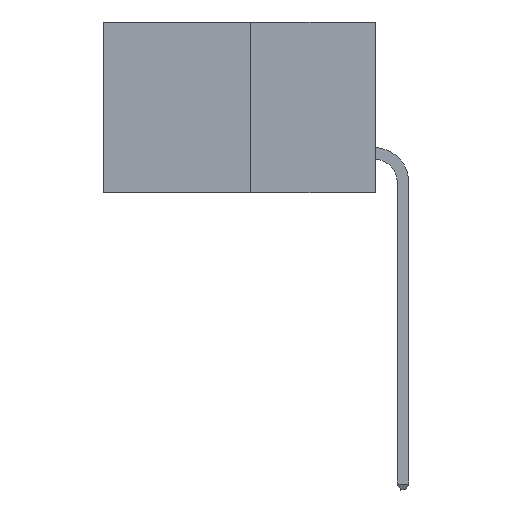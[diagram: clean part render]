
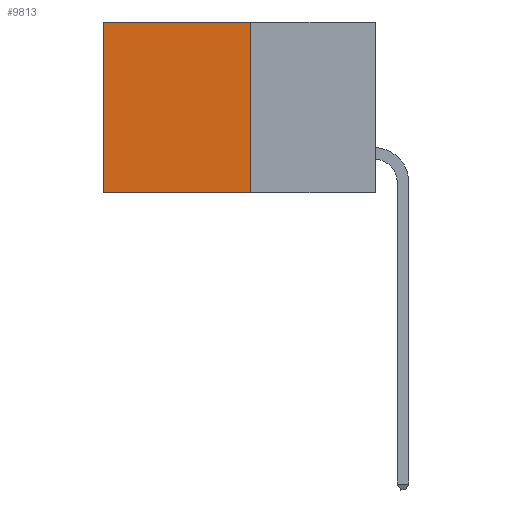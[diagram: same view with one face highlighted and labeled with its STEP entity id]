
A CAD part, left-side view. The second image highlights one B-rep face of the part: STEP entity #9813.
In plain terms, the highlighted planar face has unit normal (-1, 0, 0).
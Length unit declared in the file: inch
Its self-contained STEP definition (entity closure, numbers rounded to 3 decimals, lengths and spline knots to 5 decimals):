
#267 = CARTESIAN_POINT ( 'NONE',  ( 0.277, 0.27, 0. ) ) ;
#365 = ORIENTED_EDGE ( 'NONE', *, *, #638, .F. ) ;
#592 = CARTESIAN_POINT ( 'NONE',  ( 0.277, 0.27, -0.37 ) ) ;
#638 = EDGE_CURVE ( 'NONE', #8332, #10206, #4727, .T. ) ;
#952 = CARTESIAN_POINT ( 'NONE',  ( 0.277, 0.27, -0.37 ) ) ;
#1009 = DIRECTION ( 'NONE',  ( 0., 0., -1. ) ) ;
#1512 = VECTOR ( 'NONE', #13848, 39.37008 ) ;
#1978 = EDGE_LOOP ( 'NONE', ( #10787, #11857, #365, #2733 ) ) ;
#2433 = VECTOR ( 'NONE', #6500, 39.37008 ) ;
#2733 = ORIENTED_EDGE ( 'NONE', *, *, #5986, .T. ) ;
#3197 = VECTOR ( 'NONE', #8444, 39.37008 ) ;
#4685 = AXIS2_PLACEMENT_3D ( 'NONE', #952, #7976, #1009 ) ;
#4727 = LINE ( 'NONE', #12705, #1512 ) ;
#4744 = CARTESIAN_POINT ( 'NONE',  ( 0.277, 0.27, 0. ) ) ;
#5880 = VECTOR ( 'NONE', #8704, 39.37008 ) ;
#5986 = EDGE_CURVE ( 'NONE', #8332, #9341, #9114, .T. ) ;
#6009 = CARTESIAN_POINT ( 'NONE',  ( 0.277, 0.59, 0. ) ) ;
#6500 = DIRECTION ( 'NONE',  ( 0., 0., -1. ) ) ;
#7284 = EDGE_CURVE ( 'NONE', #10206, #7941, #8459, .T. ) ;
#7289 = EDGE_CURVE ( 'NONE', #9341, #7941, #14217, .T. ) ;
#7495 = CARTESIAN_POINT ( 'NONE',  ( 0.277, 0.59, -0.37 ) ) ;
#7941 = VERTEX_POINT ( 'NONE', #7495 ) ;
#7976 = DIRECTION ( 'NONE',  ( 1., 0., 0. ) ) ;
#8332 = VERTEX_POINT ( 'NONE', #4744 ) ;
#8444 = DIRECTION ( 'NONE',  ( 0., 1., 0. ) ) ;
#8459 = LINE ( 'NONE', #592, #5880 ) ;
#8704 = DIRECTION ( 'NONE',  ( 0., 1., 0. ) ) ;
#9114 = LINE ( 'NONE', #267, #3197 ) ;
#9341 = VERTEX_POINT ( 'NONE', #6009 ) ;
#9813 = ADVANCED_FACE ( 'NONE', ( #14477 ), #14429, .F. ) ;
#10206 = VERTEX_POINT ( 'NONE', #12815 ) ;
#10787 = ORIENTED_EDGE ( 'NONE', *, *, #7289, .T. ) ;
#11857 = ORIENTED_EDGE ( 'NONE', *, *, #7284, .F. ) ;
#12705 = CARTESIAN_POINT ( 'NONE',  ( 0.277, 0.27, -0.37 ) ) ;
#12815 = CARTESIAN_POINT ( 'NONE',  ( 0.277, 0.27, -0.37 ) ) ;
#13848 = DIRECTION ( 'NONE',  ( 0., 0., -1. ) ) ;
#14101 = CARTESIAN_POINT ( 'NONE',  ( 0.277, 0.59, -0.37 ) ) ;
#14217 = LINE ( 'NONE', #14101, #2433 ) ;
#14429 = PLANE ( 'NONE',  #4685 ) ;
#14477 = FACE_OUTER_BOUND ( 'NONE', #1978, .T. ) ;
